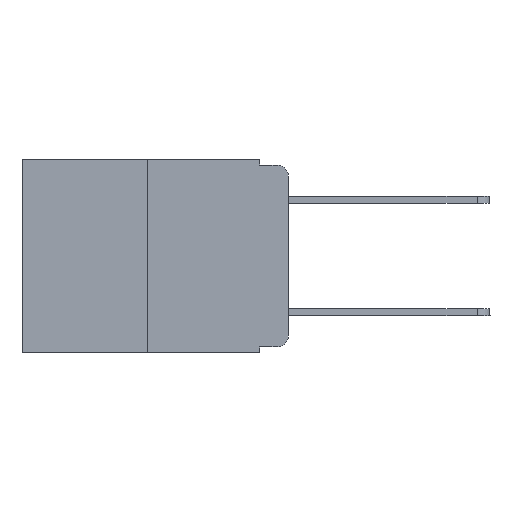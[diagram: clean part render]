
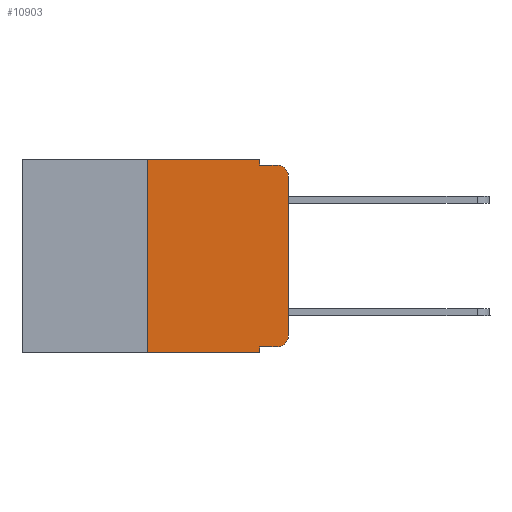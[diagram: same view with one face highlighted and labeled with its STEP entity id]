
A CAD part, left-side view. The second image highlights one B-rep face of the part: STEP entity #10903.
In plain terms, the highlighted planar face has unit normal (-1, 0, 0).
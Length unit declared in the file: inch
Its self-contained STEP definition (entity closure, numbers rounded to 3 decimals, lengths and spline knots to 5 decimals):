
#8 = CARTESIAN_POINT ( 'NONE',  ( 0., 0.02, -0.313 ) ) ;
#32 = VECTOR ( 'NONE', #15014, 39.37008 ) ;
#147 = DIRECTION ( 'NONE',  ( 0., 0., -1. ) ) ;
#559 = DIRECTION ( 'NONE',  ( 0., -1., 0. ) ) ;
#846 = EDGE_LOOP ( 'NONE', ( #8453, #2693, #16143, #15379, #13843, #5711, #5721, #7791, #5361, #16610 ) ) ;
#1008 = CARTESIAN_POINT ( 'NONE',  ( 0., 0., -0.313 ) ) ;
#2274 = CARTESIAN_POINT ( 'NONE',  ( 0., 0.02, -0.01 ) ) ;
#2526 = CARTESIAN_POINT ( 'NONE',  ( 0., 0.473, -0.343 ) ) ;
#2693 = ORIENTED_EDGE ( 'NONE', *, *, #6654, .T. ) ;
#2878 = LINE ( 'NONE', #6903, #6480 ) ;
#2915 = AXIS2_PLACEMENT_3D ( 'NONE', #15031, #16279, #4642 ) ;
#3024 = VERTEX_POINT ( 'NONE', #6443 ) ;
#3049 = EDGE_CURVE ( 'NONE', #8636, #13294, #3943, .T. ) ;
#3198 = DIRECTION ( 'NONE',  ( 0., -1., 0. ) ) ;
#3266 = CIRCLE ( 'NONE', #13485, 0.02 ) ;
#3348 = DIRECTION ( 'NONE',  ( 0., 0., -1. ) ) ;
#3419 = LINE ( 'NONE', #14726, #13803 ) ;
#3810 = VECTOR ( 'NONE', #10090, 39.37008 ) ;
#3943 = LINE ( 'NONE', #4344, #6394 ) ;
#4130 = CARTESIAN_POINT ( 'NONE',  ( 0., 0.051, 0. ) ) ;
#4344 = CARTESIAN_POINT ( 'NONE',  ( 0., 0.25, 0. ) ) ;
#4642 = DIRECTION ( 'NONE',  ( 0., 0., -1. ) ) ;
#5289 = EDGE_CURVE ( 'NONE', #15656, #10291, #9505, .T. ) ;
#5304 = DIRECTION ( 'NONE',  ( 0., 0., -1. ) ) ;
#5361 = ORIENTED_EDGE ( 'NONE', *, *, #12623, .T. ) ;
#5711 = ORIENTED_EDGE ( 'NONE', *, *, #3049, .F. ) ;
#5721 = ORIENTED_EDGE ( 'NONE', *, *, #14030, .T. ) ;
#5960 = CARTESIAN_POINT ( 'NONE',  ( 0., 0.051, -0.333 ) ) ;
#6394 = VECTOR ( 'NONE', #8304, 39.37008 ) ;
#6443 = CARTESIAN_POINT ( 'NONE',  ( 0., 0.051, -0.01 ) ) ;
#6480 = VECTOR ( 'NONE', #3198, 39.37008 ) ;
#6654 = EDGE_CURVE ( 'NONE', #10291, #11466, #15412, .T. ) ;
#6903 = CARTESIAN_POINT ( 'NONE',  ( 0., 0.473, 0. ) ) ;
#7017 = CARTESIAN_POINT ( 'NONE',  ( 0., 0.051, 0. ) ) ;
#7723 = CARTESIAN_POINT ( 'NONE',  ( 0., 0.051, -0.333 ) ) ;
#7791 = ORIENTED_EDGE ( 'NONE', *, *, #14478, .F. ) ;
#8006 = CARTESIAN_POINT ( 'NONE',  ( 0., 0.051, -0.343 ) ) ;
#8304 = DIRECTION ( 'NONE',  ( 0., 0., 1. ) ) ;
#8453 = ORIENTED_EDGE ( 'NONE', *, *, #5289, .T. ) ;
#8636 = VERTEX_POINT ( 'NONE', #10449 ) ;
#8685 = FACE_OUTER_BOUND ( 'NONE', #846, .T. ) ;
#8979 = CARTESIAN_POINT ( 'NONE',  ( 0., 0.051, 0. ) ) ;
#9095 = EDGE_CURVE ( 'NONE', #15223, #15656, #3266, .T. ) ;
#9261 = EDGE_CURVE ( 'NONE', #13294, #11302, #2878, .T. ) ;
#9484 = VERTEX_POINT ( 'NONE', #7723 ) ;
#9505 = LINE ( 'NONE', #14756, #32 ) ;
#9534 = CARTESIAN_POINT ( 'NONE',  ( 0., 0., -0.03 ) ) ;
#9691 = EDGE_CURVE ( 'NONE', #3024, #11466, #3419, .T. ) ;
#9705 = DIRECTION ( 'NONE',  ( 0., 0., -1. ) ) ;
#9782 = VECTOR ( 'NONE', #9705, 39.37008 ) ;
#10090 = DIRECTION ( 'NONE',  ( 0., -1., 0. ) ) ;
#10291 = VERTEX_POINT ( 'NONE', #9534 ) ;
#10449 = CARTESIAN_POINT ( 'NONE',  ( 0., 0.25, -0.343 ) ) ;
#10516 = VECTOR ( 'NONE', #147, 39.37008 ) ;
#10816 = AXIS2_PLACEMENT_3D ( 'NONE', #13533, #10991, #3348 ) ;
#10903 = ADVANCED_FACE ( 'NONE', ( #8685 ), #13578, .F. ) ;
#10991 = DIRECTION ( 'NONE',  ( -1., 0., 0. ) ) ;
#11191 = LINE ( 'NONE', #5960, #14831 ) ;
#11255 = VERTEX_POINT ( 'NONE', #8006 ) ;
#11284 = CARTESIAN_POINT ( 'NONE',  ( 0., 0.02, -0.333 ) ) ;
#11302 = VERTEX_POINT ( 'NONE', #4130 ) ;
#11466 = VERTEX_POINT ( 'NONE', #2274 ) ;
#11730 = EDGE_CURVE ( 'NONE', #11302, #3024, #15810, .T. ) ;
#12379 = DIRECTION ( 'NONE',  ( 0., -1., 0. ) ) ;
#12623 = EDGE_CURVE ( 'NONE', #9484, #15223, #11191, .T. ) ;
#12738 = DIRECTION ( 'NONE',  ( -1., 0., 0. ) ) ;
#13294 = VERTEX_POINT ( 'NONE', #14209 ) ;
#13485 = AXIS2_PLACEMENT_3D ( 'NONE', #8, #12738, #5304 ) ;
#13533 = CARTESIAN_POINT ( 'NONE',  ( 0., 0.02, -0.03 ) ) ;
#13578 = PLANE ( 'NONE',  #2915 ) ;
#13803 = VECTOR ( 'NONE', #559, 39.37008 ) ;
#13843 = ORIENTED_EDGE ( 'NONE', *, *, #9261, .F. ) ;
#14030 = EDGE_CURVE ( 'NONE', #8636, #11255, #16596, .T. ) ;
#14131 = LINE ( 'NONE', #8979, #10516 ) ;
#14209 = CARTESIAN_POINT ( 'NONE',  ( 0., 0.25, 0. ) ) ;
#14478 = EDGE_CURVE ( 'NONE', #9484, #11255, #14131, .T. ) ;
#14726 = CARTESIAN_POINT ( 'NONE',  ( 0., 0.051, -0.01 ) ) ;
#14756 = CARTESIAN_POINT ( 'NONE',  ( 0., 0., 0. ) ) ;
#14831 = VECTOR ( 'NONE', #12379, 39.37008 ) ;
#15014 = DIRECTION ( 'NONE',  ( 0., 0., 1. ) ) ;
#15031 = CARTESIAN_POINT ( 'NONE',  ( 0., 0.473, 0. ) ) ;
#15223 = VERTEX_POINT ( 'NONE', #11284 ) ;
#15379 = ORIENTED_EDGE ( 'NONE', *, *, #11730, .F. ) ;
#15412 = CIRCLE ( 'NONE', #10816, 0.02 ) ;
#15656 = VERTEX_POINT ( 'NONE', #1008 ) ;
#15810 = LINE ( 'NONE', #7017, #9782 ) ;
#16143 = ORIENTED_EDGE ( 'NONE', *, *, #9691, .F. ) ;
#16279 = DIRECTION ( 'NONE',  ( 1., 0., 0. ) ) ;
#16596 = LINE ( 'NONE', #2526, #3810 ) ;
#16610 = ORIENTED_EDGE ( 'NONE', *, *, #9095, .T. ) ;
